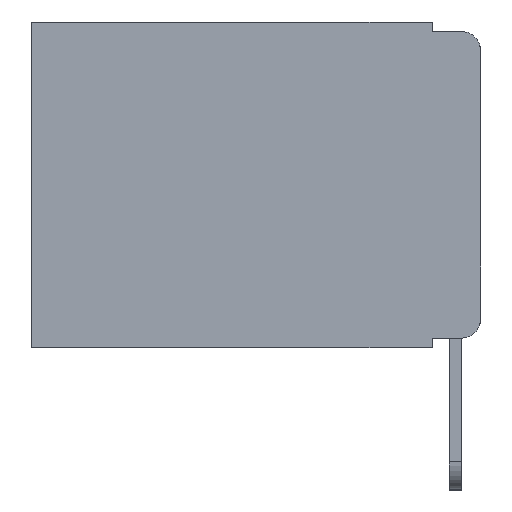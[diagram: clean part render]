
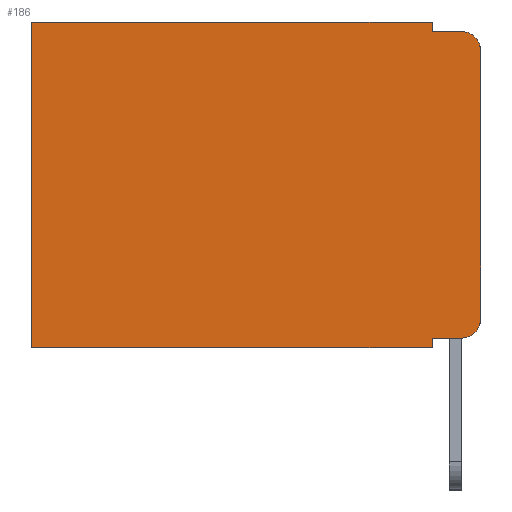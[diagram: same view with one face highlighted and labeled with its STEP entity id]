
A CAD part, left-side view. The second image highlights one B-rep face of the part: STEP entity #186.
In plain terms, the highlighted planar face has unit normal (-1, 0, 0).
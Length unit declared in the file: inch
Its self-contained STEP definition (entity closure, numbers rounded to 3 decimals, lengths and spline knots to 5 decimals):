
#157 = EDGE_CURVE ( 'NONE', #12635, #9111, #5498, .T. ) ;
#186 = ADVANCED_FACE ( 'NONE', ( #12505 ), #15020, .F. ) ;
#246 = VECTOR ( 'NONE', #16480, 39.37008 ) ;
#263 = CARTESIAN_POINT ( 'NONE',  ( 0.298, 0., 0. ) ) ;
#344 = EDGE_CURVE ( 'NONE', #7587, #12891, #11057, .T. ) ;
#606 = CARTESIAN_POINT ( 'NONE',  ( 0.298, 0., -0.313 ) ) ;
#822 = AXIS2_PLACEMENT_3D ( 'NONE', #5522, #4166, #2680 ) ;
#908 = CARTESIAN_POINT ( 'NONE',  ( 0.298, 0.051, -0.343 ) ) ;
#936 = LINE ( 'NONE', #3816, #10114 ) ;
#1138 = DIRECTION ( 'NONE',  ( 0., 0., -1. ) ) ;
#1347 = DIRECTION ( 'NONE',  ( 0., 0., -1. ) ) ;
#1387 = CARTESIAN_POINT ( 'NONE',  ( 0.298, 0., 0. ) ) ;
#1615 = CARTESIAN_POINT ( 'NONE',  ( 0.298, 0.473, -0.343 ) ) ;
#2134 = CARTESIAN_POINT ( 'NONE',  ( 0.298, 0.051, -0.333 ) ) ;
#2438 = DIRECTION ( 'NONE',  ( 0., -1., 0. ) ) ;
#2677 = CARTESIAN_POINT ( 'NONE',  ( 0.298, 0.051, 0. ) ) ;
#2680 = DIRECTION ( 'NONE',  ( 0., 0., -1. ) ) ;
#2780 = ORIENTED_EDGE ( 'NONE', *, *, #157, .F. ) ;
#2804 = CARTESIAN_POINT ( 'NONE',  ( 0.298, 0., 0. ) ) ;
#2821 = EDGE_CURVE ( 'NONE', #15003, #13793, #936, .T. ) ;
#2946 = VECTOR ( 'NONE', #13842, 39.37008 ) ;
#3144 = ORIENTED_EDGE ( 'NONE', *, *, #2821, .F. ) ;
#3228 = EDGE_CURVE ( 'NONE', #11692, #13082, #7500, .T. ) ;
#3816 = CARTESIAN_POINT ( 'NONE',  ( 0.298, 0.051, 0. ) ) ;
#4152 = DIRECTION ( 'NONE',  ( 0., 0., -1. ) ) ;
#4166 = DIRECTION ( 'NONE',  ( -1., 0., 0. ) ) ;
#4355 = ORIENTED_EDGE ( 'NONE', *, *, #13395, .F. ) ;
#5498 = LINE ( 'NONE', #1387, #7843 ) ;
#5522 = CARTESIAN_POINT ( 'NONE',  ( 0.298, 0.02, -0.313 ) ) ;
#5995 = CARTESIAN_POINT ( 'NONE',  ( 0.298, 0., -0.03 ) ) ;
#6619 = ORIENTED_EDGE ( 'NONE', *, *, #15588, .F. ) ;
#7236 = EDGE_CURVE ( 'NONE', #12635, #11455, #12130, .T. ) ;
#7500 = LINE ( 'NONE', #16648, #246 ) ;
#7587 = VERTEX_POINT ( 'NONE', #10591 ) ;
#7843 = VECTOR ( 'NONE', #4152, 39.37008 ) ;
#7920 = CARTESIAN_POINT ( 'NONE',  ( 0.298, 0.051, -0.01 ) ) ;
#8057 = DIRECTION ( 'NONE',  ( 0., 1., 0. ) ) ;
#8129 = ORIENTED_EDGE ( 'NONE', *, *, #17350, .T. ) ;
#8398 = DIRECTION ( 'NONE',  ( 0., 0., -1. ) ) ;
#8684 = VECTOR ( 'NONE', #8057, 39.37008 ) ;
#9111 = VERTEX_POINT ( 'NONE', #606 ) ;
#9359 = EDGE_CURVE ( 'NONE', #11692, #10285, #17471, .T. ) ;
#9719 = CIRCLE ( 'NONE', #822, 0.02 ) ;
#9781 = CARTESIAN_POINT ( 'NONE',  ( 0.298, 0.051, -0.01 ) ) ;
#9811 = DIRECTION ( 'NONE',  ( -1., 0., 0. ) ) ;
#10114 = VECTOR ( 'NONE', #1138, 39.37008 ) ;
#10285 = VERTEX_POINT ( 'NONE', #908 ) ;
#10288 = VECTOR ( 'NONE', #1347, 39.37008 ) ;
#10591 = CARTESIAN_POINT ( 'NONE',  ( 0.298, 0.473, 0. ) ) ;
#10667 = ORIENTED_EDGE ( 'NONE', *, *, #15789, .T. ) ;
#11057 = LINE ( 'NONE', #12926, #17379 ) ;
#11156 = VECTOR ( 'NONE', #2438, 39.37008 ) ;
#11403 = CARTESIAN_POINT ( 'NONE',  ( 0.298, 0.02, -0.01 ) ) ;
#11442 = CARTESIAN_POINT ( 'NONE',  ( 0.298, 0.02, -0.333 ) ) ;
#11455 = VERTEX_POINT ( 'NONE', #11403 ) ;
#11565 = DIRECTION ( 'NONE',  ( 0., 0., -1. ) ) ;
#11692 = VERTEX_POINT ( 'NONE', #2134 ) ;
#11990 = LINE ( 'NONE', #9781, #11156 ) ;
#12072 = CARTESIAN_POINT ( 'NONE',  ( 0.298, 0., -0.343 ) ) ;
#12130 = CIRCLE ( 'NONE', #16072, 0.02 ) ;
#12234 = ORIENTED_EDGE ( 'NONE', *, *, #344, .T. ) ;
#12505 = FACE_OUTER_BOUND ( 'NONE', #14123, .T. ) ;
#12635 = VERTEX_POINT ( 'NONE', #5995 ) ;
#12891 = VERTEX_POINT ( 'NONE', #1615 ) ;
#12926 = CARTESIAN_POINT ( 'NONE',  ( 0.298, 0.473, 0. ) ) ;
#13082 = VERTEX_POINT ( 'NONE', #11442 ) ;
#13230 = ORIENTED_EDGE ( 'NONE', *, *, #3228, .T. ) ;
#13395 = EDGE_CURVE ( 'NONE', #10285, #12891, #15676, .T. ) ;
#13527 = CARTESIAN_POINT ( 'NONE',  ( 0.298, 0.051, 0. ) ) ;
#13792 = LINE ( 'NONE', #2804, #2946 ) ;
#13793 = VERTEX_POINT ( 'NONE', #7920 ) ;
#13842 = DIRECTION ( 'NONE',  ( 0., 1., 0. ) ) ;
#13888 = CARTESIAN_POINT ( 'NONE',  ( 0.298, 0.02, -0.03 ) ) ;
#14123 = EDGE_LOOP ( 'NONE', ( #2780, #15356, #6619, #3144, #10667, #12234, #4355, #16905, #13230, #8129 ) ) ;
#15003 = VERTEX_POINT ( 'NONE', #13527 ) ;
#15020 = PLANE ( 'NONE',  #16249 ) ;
#15077 = DIRECTION ( 'NONE',  ( 1., 0., 0. ) ) ;
#15198 = DIRECTION ( 'NONE',  ( 0., 0., -1. ) ) ;
#15356 = ORIENTED_EDGE ( 'NONE', *, *, #7236, .T. ) ;
#15588 = EDGE_CURVE ( 'NONE', #13793, #11455, #11990, .T. ) ;
#15676 = LINE ( 'NONE', #12072, #8684 ) ;
#15789 = EDGE_CURVE ( 'NONE', #15003, #7587, #13792, .T. ) ;
#16072 = AXIS2_PLACEMENT_3D ( 'NONE', #13888, #9811, #15198 ) ;
#16249 = AXIS2_PLACEMENT_3D ( 'NONE', #263, #15077, #8398 ) ;
#16480 = DIRECTION ( 'NONE',  ( 0., -1., 0. ) ) ;
#16648 = CARTESIAN_POINT ( 'NONE',  ( 0.298, 0.051, -0.333 ) ) ;
#16905 = ORIENTED_EDGE ( 'NONE', *, *, #9359, .F. ) ;
#17350 = EDGE_CURVE ( 'NONE', #13082, #9111, #9719, .T. ) ;
#17379 = VECTOR ( 'NONE', #11565, 39.37008 ) ;
#17471 = LINE ( 'NONE', #2677, #10288 ) ;
